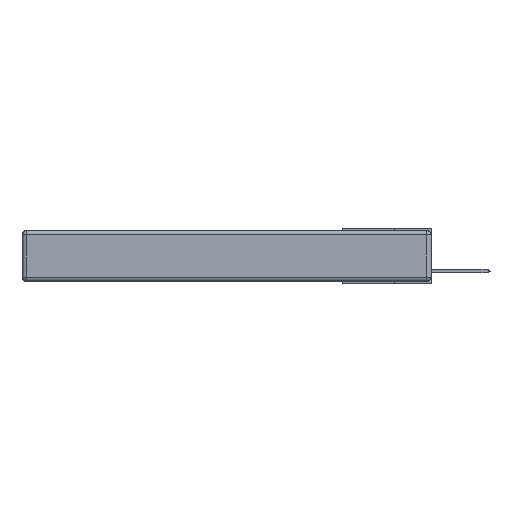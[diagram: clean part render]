
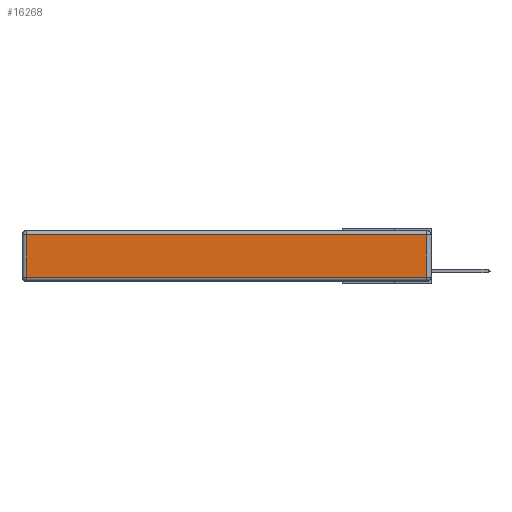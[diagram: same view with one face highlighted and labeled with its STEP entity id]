
A CAD part, left-side view. The second image highlights one B-rep face of the part: STEP entity #16268.
In plain terms, the highlighted planar face has unit normal (-1, 0, 0).
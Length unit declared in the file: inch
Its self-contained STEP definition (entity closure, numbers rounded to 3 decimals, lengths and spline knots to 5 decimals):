
#939 = VECTOR ( 'NONE', #13166, 39.37008 ) ;
#1224 = LINE ( 'NONE', #17260, #15588 ) ;
#2828 = EDGE_CURVE ( 'NONE', #22144, #4150, #12069, .T. ) ;
#4150 = VERTEX_POINT ( 'NONE', #15679 ) ;
#4356 = PLANE ( 'NONE',  #21502 ) ;
#4968 = ORIENTED_EDGE ( 'NONE', *, *, #11337, .T. ) ;
#6638 = DIRECTION ( 'NONE',  ( -1., 0., 0. ) ) ;
#7093 = ORIENTED_EDGE ( 'NONE', *, *, #26310, .T. ) ;
#7120 = ORIENTED_EDGE ( 'NONE', *, *, #21515, .T. ) ;
#8010 = CARTESIAN_POINT ( 'NONE',  ( 0., 2.72, -0.313 ) ) ;
#9653 = VECTOR ( 'NONE', #17058, 39.37008 ) ;
#10674 = ORIENTED_EDGE ( 'NONE', *, *, #2828, .T. ) ;
#10734 = CARTESIAN_POINT ( 'NONE',  ( 0., 0.03, -0.313 ) ) ;
#11337 = EDGE_CURVE ( 'NONE', #4150, #13380, #1224, .T. ) ;
#12069 = LINE ( 'NONE', #29096, #939 ) ;
#12596 = CARTESIAN_POINT ( 'NONE',  ( 0., 0., -0.313 ) ) ;
#13166 = DIRECTION ( 'NONE',  ( 0., 1., 0. ) ) ;
#13380 = VERTEX_POINT ( 'NONE', #8010 ) ;
#13544 = DIRECTION ( 'NONE',  ( 0., 0., 1. ) ) ;
#13717 = DIRECTION ( 'NONE',  ( 0., 0., 1. ) ) ;
#14794 = VECTOR ( 'NONE', #13717, 39.37008 ) ;
#15588 = VECTOR ( 'NONE', #22015, 39.37008 ) ;
#15679 = CARTESIAN_POINT ( 'NONE',  ( 0., 2.72, -0.03 ) ) ;
#15751 = LINE ( 'NONE', #12596, #9653 ) ;
#16268 = ADVANCED_FACE ( 'NONE', ( #22046 ), #4356, .T. ) ;
#16819 = VERTEX_POINT ( 'NONE', #10734 ) ;
#17058 = DIRECTION ( 'NONE',  ( 0., -1., 0. ) ) ;
#17260 = CARTESIAN_POINT ( 'NONE',  ( 0., 2.72, -0.343 ) ) ;
#21502 = AXIS2_PLACEMENT_3D ( 'NONE', #22544, #6638, #13544 ) ;
#21515 = EDGE_CURVE ( 'NONE', #13380, #16819, #15751, .T. ) ;
#22015 = DIRECTION ( 'NONE',  ( 0., 0., -1. ) ) ;
#22046 = FACE_OUTER_BOUND ( 'NONE', #28178, .T. ) ;
#22144 = VERTEX_POINT ( 'NONE', #23367 ) ;
#22544 = CARTESIAN_POINT ( 'NONE',  ( 0., 0., -0.343 ) ) ;
#23367 = CARTESIAN_POINT ( 'NONE',  ( 0., 0.03, -0.03 ) ) ;
#26310 = EDGE_CURVE ( 'NONE', #16819, #22144, #28026, .T. ) ;
#27220 = CARTESIAN_POINT ( 'NONE',  ( 0., 0.03, -0.343 ) ) ;
#28026 = LINE ( 'NONE', #27220, #14794 ) ;
#28178 = EDGE_LOOP ( 'NONE', ( #7120, #7093, #10674, #4968 ) ) ;
#29096 = CARTESIAN_POINT ( 'NONE',  ( 0., 2.75, -0.03 ) ) ;
